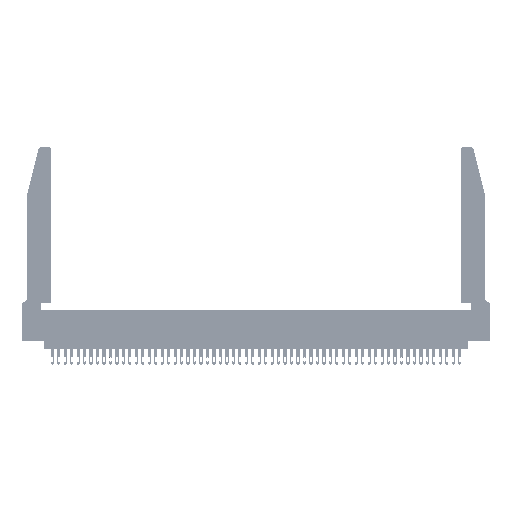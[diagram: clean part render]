
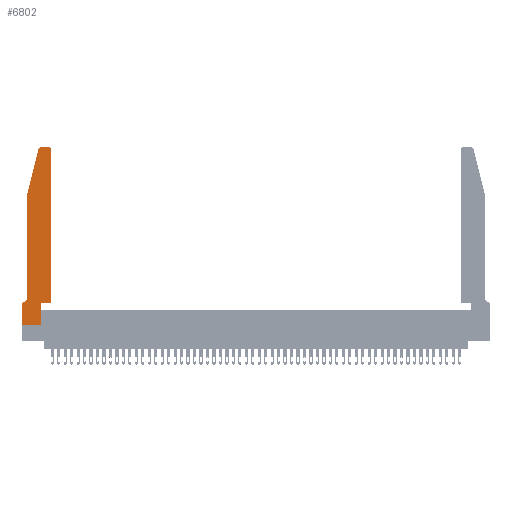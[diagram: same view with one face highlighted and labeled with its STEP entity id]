
A CAD part, top view. The second image highlights one B-rep face of the part: STEP entity #6802.
In plain terms, the highlighted planar face has unit normal (0, 0, 1).
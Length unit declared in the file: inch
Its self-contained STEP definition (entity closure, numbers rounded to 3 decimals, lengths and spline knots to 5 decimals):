
#1695 = ORIENTED_EDGE ( 'NONE', *, *, #31892, .T. ) ;
#1987 = CARTESIAN_POINT ( 'NONE',  ( 0.0755, 0.42, 0.37 ) ) ;
#2944 = CIRCLE ( 'NONE', #50354, 0.03 ) ;
#3797 = LINE ( 'NONE', #7826, #49094 ) ;
#5201 = ORIENTED_EDGE ( 'NONE', *, *, #31654, .T. ) ;
#5558 = DIRECTION ( 'NONE',  ( 1., 0., 0. ) ) ;
#5841 = CARTESIAN_POINT ( 'NONE',  ( 0.2865, 0.35, 0.37 ) ) ;
#6256 = VECTOR ( 'NONE', #38962, 39.37008 ) ;
#6802 = ADVANCED_FACE ( 'NONE', ( #27738 ), #46543, .T. ) ;
#7005 = VECTOR ( 'NONE', #42110, 39.37008 ) ;
#7425 = VERTEX_POINT ( 'NONE', #40621 ) ;
#7746 = ORIENTED_EDGE ( 'NONE', *, *, #21142, .T. ) ;
#7826 = CARTESIAN_POINT ( 'NONE',  ( 0.4505, 0.35, 0.37 ) ) ;
#8257 = EDGE_CURVE ( 'NONE', #31329, #7425, #32082, .T. ) ;
#8456 = EDGE_CURVE ( 'NONE', #26328, #46782, #17535, .T. ) ;
#10484 = AXIS2_PLACEMENT_3D ( 'NONE', #17822, #26093, #38596 ) ;
#12151 = DIRECTION ( 'NONE',  ( 0., 1., 0. ) ) ;
#12654 = DIRECTION ( 'NONE',  ( 0., -1., 0. ) ) ;
#12735 = CARTESIAN_POINT ( 'NONE',  ( 0.0755, 0.35, 0.37 ) ) ;
#13611 = CARTESIAN_POINT ( 'NONE',  ( 0.0055, 0.42, 0.37 ) ) ;
#14815 = CARTESIAN_POINT ( 'NONE',  ( 0.0055, 0.35, 0.37 ) ) ;
#15464 = ORIENTED_EDGE ( 'NONE', *, *, #15730, .T. ) ;
#15730 = EDGE_CURVE ( 'NONE', #22607, #34297, #47616, .T. ) ;
#17083 = VECTOR ( 'NONE', #12151, 39.37008 ) ;
#17535 = LINE ( 'NONE', #30874, #6256 ) ;
#17675 = DIRECTION ( 'NONE',  ( 0., 0., 1. ) ) ;
#17822 = CARTESIAN_POINT ( 'NONE',  ( 0., 0.35, 0.37 ) ) ;
#19833 = ORIENTED_EDGE ( 'NONE', *, *, #51359, .T. ) ;
#19875 = ORIENTED_EDGE ( 'NONE', *, *, #8456, .T. ) ;
#20094 = VECTOR ( 'NONE', #45137, 39.37008 ) ;
#20198 = VECTOR ( 'NONE', #34682, 39.37008 ) ;
#20394 = CARTESIAN_POINT ( 'NONE',  ( 0.4505, 0.35, 0.37 ) ) ;
#21142 = EDGE_CURVE ( 'NONE', #31293, #33033, #50578, .T. ) ;
#21458 = LINE ( 'NONE', #5841, #7005 ) ;
#21513 = LINE ( 'NONE', #43309, #20198 ) ;
#21691 = CARTESIAN_POINT ( 'NONE',  ( 0.25487, 2.72718, 0.37 ) ) ;
#22145 = VERTEX_POINT ( 'NONE', #39202 ) ;
#22400 = VERTEX_POINT ( 'NONE', #21691 ) ;
#22420 = EDGE_CURVE ( 'NONE', #46782, #22400, #48929, .T. ) ;
#22607 = VERTEX_POINT ( 'NONE', #23768 ) ;
#23768 = CARTESIAN_POINT ( 'NONE',  ( 0., 0., 0.37 ) ) ;
#23828 = LINE ( 'NONE', #39478, #33296 ) ;
#24290 = CARTESIAN_POINT ( 'NONE',  ( 0.4505, 0.35, 0.37 ) ) ;
#24486 = CARTESIAN_POINT ( 'NONE',  ( 0.4205, 2.72, 0.37 ) ) ;
#25734 = ORIENTED_EDGE ( 'NONE', *, *, #45979, .T. ) ;
#25930 = CARTESIAN_POINT ( 'NONE',  ( 0.284, 2.72, 0.37 ) ) ;
#26093 = DIRECTION ( 'NONE',  ( 0., 0., 1. ) ) ;
#26328 = VERTEX_POINT ( 'NONE', #44947 ) ;
#27088 = ORIENTED_EDGE ( 'NONE', *, *, #38427, .T. ) ;
#27286 = VERTEX_POINT ( 'NONE', #34819 ) ;
#27604 = CARTESIAN_POINT ( 'NONE',  ( 0.2865, 0., 0.37 ) ) ;
#27738 = FACE_OUTER_BOUND ( 'NONE', #41839, .T. ) ;
#30090 = ORIENTED_EDGE ( 'NONE', *, *, #8257, .T. ) ;
#30874 = CARTESIAN_POINT ( 'NONE',  ( 0.2605, 2.75, 0.37 ) ) ;
#31293 = VERTEX_POINT ( 'NONE', #37909 ) ;
#31329 = VERTEX_POINT ( 'NONE', #14815 ) ;
#31654 = EDGE_CURVE ( 'NONE', #48579, #27286, #46087, .T. ) ;
#31892 = EDGE_CURVE ( 'NONE', #34297, #22145, #21458, .T. ) ;
#31917 = DIRECTION ( 'NONE',  ( 1., 0., 0. ) ) ;
#32017 = EDGE_CURVE ( 'NONE', #22400, #31293, #21513, .T. ) ;
#32082 = LINE ( 'NONE', #12735, #20094 ) ;
#32692 = ORIENTED_EDGE ( 'NONE', *, *, #51964, .T. ) ;
#32871 = CARTESIAN_POINT ( 'NONE',  ( 0.0755, 2., 0.37 ) ) ;
#33033 = VERTEX_POINT ( 'NONE', #1987 ) ;
#33296 = VECTOR ( 'NONE', #35774, 39.37008 ) ;
#33517 = AXIS2_PLACEMENT_3D ( 'NONE', #25930, #17675, #5558 ) ;
#34280 = ORIENTED_EDGE ( 'NONE', *, *, #22420, .T. ) ;
#34297 = VERTEX_POINT ( 'NONE', #27604 ) ;
#34682 = DIRECTION ( 'NONE',  ( -0.239, -0.971, 0. ) ) ;
#34819 = CARTESIAN_POINT ( 'NONE',  ( 0.4505, 2.72, 0.37 ) ) ;
#35774 = DIRECTION ( 'NONE',  ( 0., -1., 0. ) ) ;
#36118 = DIRECTION ( 'NONE',  ( 0., 0., 1. ) ) ;
#36916 = VECTOR ( 'NONE', #39855, 39.37008 ) ;
#37909 = CARTESIAN_POINT ( 'NONE',  ( 0.0755, 2., 0.37 ) ) ;
#38055 = ORIENTED_EDGE ( 'NONE', *, *, #32017, .T. ) ;
#38427 = EDGE_CURVE ( 'NONE', #33033, #31329, #44318, .T. ) ;
#38596 = DIRECTION ( 'NONE',  ( 1., 0., 0. ) ) ;
#38962 = DIRECTION ( 'NONE',  ( -1., 0., 0. ) ) ;
#39202 = CARTESIAN_POINT ( 'NONE',  ( 0.2865, 0.35, 0.37 ) ) ;
#39478 = CARTESIAN_POINT ( 'NONE',  ( 0., 0., 0.37 ) ) ;
#39525 = CARTESIAN_POINT ( 'NONE',  ( 0., 0., 0.37 ) ) ;
#39855 = DIRECTION ( 'NONE',  ( 1., 0., 0. ) ) ;
#40562 = DIRECTION ( 'NONE',  ( 1., 0., 0. ) ) ;
#40621 = CARTESIAN_POINT ( 'NONE',  ( 0., 0.35, 0.37 ) ) ;
#41269 = DIRECTION ( 'NONE',  ( 0., 0., -1. ) ) ;
#41839 = EDGE_LOOP ( 'NONE', ( #19875, #34280, #38055, #7746, #27088, #30090, #32692, #15464, #1695, #19833, #5201, #25734 ) ) ;
#42110 = DIRECTION ( 'NONE',  ( 0., 1., 0. ) ) ;
#42452 = VECTOR ( 'NONE', #12654, 39.37008 ) ;
#43091 = AXIS2_PLACEMENT_3D ( 'NONE', #13611, #41269, #49317 ) ;
#43270 = CARTESIAN_POINT ( 'NONE',  ( 0.284, 2.75, 0.37 ) ) ;
#43309 = CARTESIAN_POINT ( 'NONE',  ( 0.0755, 2., 0.37 ) ) ;
#44318 = CIRCLE ( 'NONE', #43091, 0.07 ) ;
#44947 = CARTESIAN_POINT ( 'NONE',  ( 0.4205, 2.75, 0.37 ) ) ;
#45137 = DIRECTION ( 'NONE',  ( -1., 0., 0. ) ) ;
#45979 = EDGE_CURVE ( 'NONE', #27286, #26328, #2944, .T. ) ;
#46087 = LINE ( 'NONE', #20394, #17083 ) ;
#46543 = PLANE ( 'NONE',  #10484 ) ;
#46782 = VERTEX_POINT ( 'NONE', #43270 ) ;
#47616 = LINE ( 'NONE', #39525, #36916 ) ;
#48579 = VERTEX_POINT ( 'NONE', #24290 ) ;
#48929 = CIRCLE ( 'NONE', #33517, 0.03 ) ;
#49094 = VECTOR ( 'NONE', #40562, 39.37008 ) ;
#49317 = DIRECTION ( 'NONE',  ( -1., 0., 0. ) ) ;
#50354 = AXIS2_PLACEMENT_3D ( 'NONE', #24486, #36118, #31917 ) ;
#50578 = LINE ( 'NONE', #32871, #42452 ) ;
#51359 = EDGE_CURVE ( 'NONE', #22145, #48579, #3797, .T. ) ;
#51964 = EDGE_CURVE ( 'NONE', #7425, #22607, #23828, .T. ) ;
